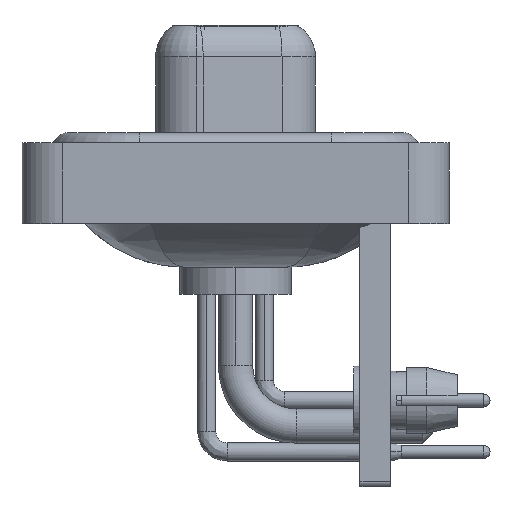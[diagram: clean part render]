
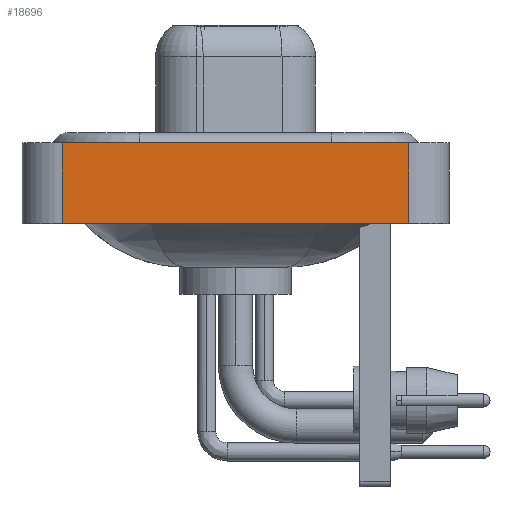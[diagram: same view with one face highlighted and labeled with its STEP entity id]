
A CAD part, left-side view. The second image highlights one B-rep face of the part: STEP entity #18696.
In plain terms, the highlighted planar face has unit normal (-1, 0, 0).
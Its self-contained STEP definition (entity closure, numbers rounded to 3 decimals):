
#216 = DIRECTION ( 'NONE',  ( 0., -1., 0. ) ) ;
#483 = CARTESIAN_POINT ( 'NONE',  ( -7.3, 8.55, 0.4 ) ) ;
#1724 = LINE ( 'NONE', #15980, #7056 ) ;
#2111 = EDGE_CURVE ( 'NONE', #14882, #6292, #15592, .T. ) ;
#2163 = EDGE_LOOP ( 'NONE', ( #17132, #5477, #14891, #22656 ) ) ;
#3392 = EDGE_CURVE ( 'NONE', #16228, #6292, #8738, .T. ) ;
#3584 = CARTESIAN_POINT ( 'NONE',  ( -7.3, -8.55, -3.6 ) ) ;
#3997 = AXIS2_PLACEMENT_3D ( 'NONE', #19076, #10208, #17340 ) ;
#4857 = PLANE ( 'NONE',  #3997 ) ;
#5322 = VECTOR ( 'NONE', #14413, 1000. ) ;
#5477 = ORIENTED_EDGE ( 'NONE', *, *, #3392, .F. ) ;
#6268 = EDGE_CURVE ( 'NONE', #23046, #16228, #11015, .T. ) ;
#6292 = VERTEX_POINT ( 'NONE', #14857 ) ;
#7056 = VECTOR ( 'NONE', #216, 1000. ) ;
#8738 = LINE ( 'NONE', #17289, #20713 ) ;
#10208 = DIRECTION ( 'NONE',  ( -1., 0., 0. ) ) ;
#10985 = CARTESIAN_POINT ( 'NONE',  ( -7.3, -8.55, -3.6 ) ) ;
#11015 = LINE ( 'NONE', #19766, #5322 ) ;
#14079 = DIRECTION ( 'NONE',  ( 0., 0., 1. ) ) ;
#14413 = DIRECTION ( 'NONE',  ( 0., 0., 1. ) ) ;
#14857 = CARTESIAN_POINT ( 'NONE',  ( -7.3, -8.55, 0.4 ) ) ;
#14882 = VERTEX_POINT ( 'NONE', #10985 ) ;
#14891 = ORIENTED_EDGE ( 'NONE', *, *, #6268, .F. ) ;
#15179 = VECTOR ( 'NONE', #14079, 1000. ) ;
#15592 = LINE ( 'NONE', #3584, #15179 ) ;
#15980 = CARTESIAN_POINT ( 'NONE',  ( -7.3, -8.55, -3.6 ) ) ;
#16228 = VERTEX_POINT ( 'NONE', #483 ) ;
#17132 = ORIENTED_EDGE ( 'NONE', *, *, #2111, .T. ) ;
#17289 = CARTESIAN_POINT ( 'NONE',  ( -7.3, -8.55, 0.4 ) ) ;
#17340 = DIRECTION ( 'NONE',  ( 0., 0., 1. ) ) ;
#18389 = EDGE_CURVE ( 'NONE', #23046, #14882, #1724, .T. ) ;
#18696 = ADVANCED_FACE ( 'NONE', ( #20841 ), #4857, .T. ) ;
#19076 = CARTESIAN_POINT ( 'NONE',  ( -7.3, -8.55, -3.6 ) ) ;
#19337 = CARTESIAN_POINT ( 'NONE',  ( -7.3, 8.55, -3.6 ) ) ;
#19766 = CARTESIAN_POINT ( 'NONE',  ( -7.3, 8.55, -3.6 ) ) ;
#20713 = VECTOR ( 'NONE', #21262, 1000. ) ;
#20841 = FACE_OUTER_BOUND ( 'NONE', #2163, .T. ) ;
#21262 = DIRECTION ( 'NONE',  ( 0., -1., 0. ) ) ;
#22656 = ORIENTED_EDGE ( 'NONE', *, *, #18389, .T. ) ;
#23046 = VERTEX_POINT ( 'NONE', #19337 ) ;
